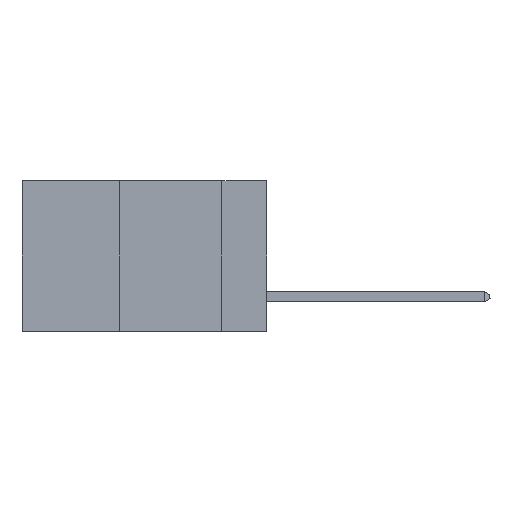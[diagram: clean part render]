
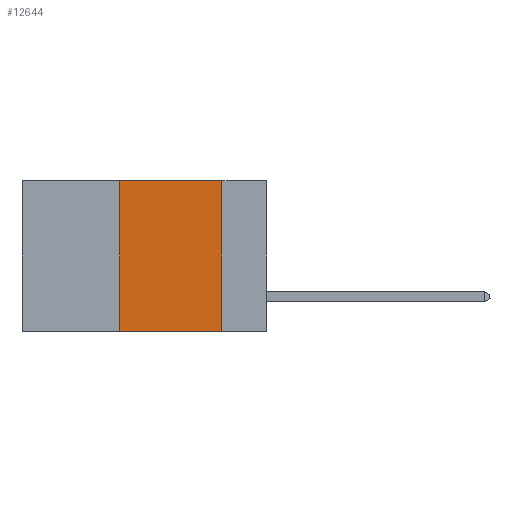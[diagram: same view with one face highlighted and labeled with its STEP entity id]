
A CAD part, left-side view. The second image highlights one B-rep face of the part: STEP entity #12644.
In plain terms, the highlighted planar face has unit normal (-1, 0, 0).
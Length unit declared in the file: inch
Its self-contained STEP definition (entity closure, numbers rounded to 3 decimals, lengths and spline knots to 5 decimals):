
#34 = CARTESIAN_POINT ( 'NONE',  ( 0., 0.6, 0. ) ) ;
#89 = CARTESIAN_POINT ( 'NONE',  ( 0., 0.36, 0. ) ) ;
#543 = LINE ( 'NONE', #89, #1312 ) ;
#975 = ORIENTED_EDGE ( 'NONE', *, *, #12681, .F. ) ;
#1312 = VECTOR ( 'NONE', #8332, 39.37008 ) ;
#1381 = CARTESIAN_POINT ( 'NONE',  ( 0., 0.36, -0.37 ) ) ;
#1681 = ORIENTED_EDGE ( 'NONE', *, *, #12256, .F. ) ;
#2013 = DIRECTION ( 'NONE',  ( 0., -1., 0. ) ) ;
#2237 = CARTESIAN_POINT ( 'NONE',  ( 0., 0.11, -0.37 ) ) ;
#2663 = LINE ( 'NONE', #4179, #15544 ) ;
#3200 = VECTOR ( 'NONE', #2013, 39.37008 ) ;
#3428 = CARTESIAN_POINT ( 'NONE',  ( 0., 0.6, 0. ) ) ;
#3685 = DIRECTION ( 'NONE',  ( 0., 0., -1. ) ) ;
#3909 = AXIS2_PLACEMENT_3D ( 'NONE', #34, #9683, #3685 ) ;
#3966 = DIRECTION ( 'NONE',  ( 0., 0., -1. ) ) ;
#4179 = CARTESIAN_POINT ( 'NONE',  ( 0., 0.11, 0. ) ) ;
#4347 = EDGE_CURVE ( 'NONE', #5533, #6608, #14207, .T. ) ;
#4474 = VERTEX_POINT ( 'NONE', #13200 ) ;
#5533 = VERTEX_POINT ( 'NONE', #1381 ) ;
#5766 = DIRECTION ( 'NONE',  ( 0., -1., 0. ) ) ;
#6608 = VERTEX_POINT ( 'NONE', #2237 ) ;
#6792 = FACE_OUTER_BOUND ( 'NONE', #13739, .T. ) ;
#6965 = CARTESIAN_POINT ( 'NONE',  ( 0., 0.6, -0.37 ) ) ;
#7741 = ORIENTED_EDGE ( 'NONE', *, *, #9839, .F. ) ;
#7827 = VECTOR ( 'NONE', #5766, 39.37008 ) ;
#8332 = DIRECTION ( 'NONE',  ( 0., 0., 1. ) ) ;
#8764 = LINE ( 'NONE', #3428, #7827 ) ;
#9683 = DIRECTION ( 'NONE',  ( 1., 0., 0. ) ) ;
#9839 = EDGE_CURVE ( 'NONE', #4474, #12375, #8764, .T. ) ;
#11085 = ORIENTED_EDGE ( 'NONE', *, *, #4347, .T. ) ;
#12256 = EDGE_CURVE ( 'NONE', #12375, #6608, #2663, .T. ) ;
#12375 = VERTEX_POINT ( 'NONE', #12836 ) ;
#12644 = ADVANCED_FACE ( 'NONE', ( #6792 ), #15610, .F. ) ;
#12681 = EDGE_CURVE ( 'NONE', #5533, #4474, #543, .T. ) ;
#12836 = CARTESIAN_POINT ( 'NONE',  ( 0., 0.11, 0. ) ) ;
#13200 = CARTESIAN_POINT ( 'NONE',  ( 0., 0.36, 0. ) ) ;
#13739 = EDGE_LOOP ( 'NONE', ( #1681, #7741, #975, #11085 ) ) ;
#14207 = LINE ( 'NONE', #6965, #3200 ) ;
#15544 = VECTOR ( 'NONE', #3966, 39.37008 ) ;
#15610 = PLANE ( 'NONE',  #3909 ) ;
